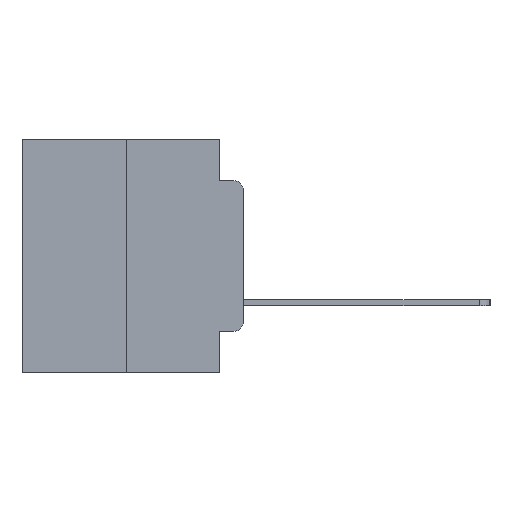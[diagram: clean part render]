
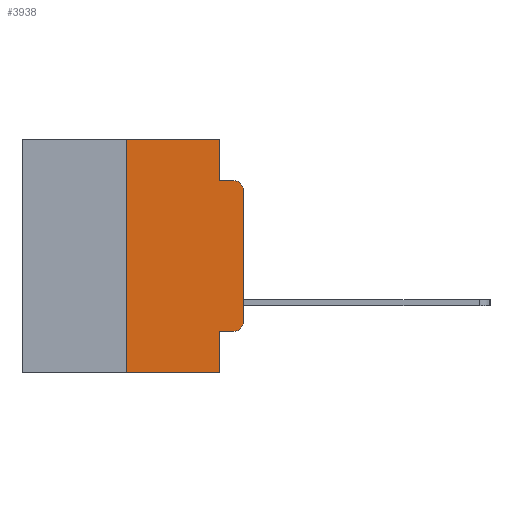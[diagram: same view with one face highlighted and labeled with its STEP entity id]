
A CAD part, left-side view. The second image highlights one B-rep face of the part: STEP entity #3938.
In plain terms, the highlighted planar face has unit normal (-1, 0, 0).
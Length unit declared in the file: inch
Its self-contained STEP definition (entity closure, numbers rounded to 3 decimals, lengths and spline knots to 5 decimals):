
#409 = DIRECTION ( 'NONE',  ( 0., 0., -1. ) ) ;
#796 = VECTOR ( 'NONE', #15762, 39.37008 ) ;
#1308 = DIRECTION ( 'NONE',  ( 0., 0., 1. ) ) ;
#1438 = DIRECTION ( 'NONE',  ( 0., -1., 0. ) ) ;
#1611 = ORIENTED_EDGE ( 'NONE', *, *, #8251, .T. ) ;
#1796 = EDGE_CURVE ( 'NONE', #16303, #14823, #22800, .T. ) ;
#1822 = AXIS2_PLACEMENT_3D ( 'NONE', #10927, #16995, #4756 ) ;
#1959 = ORIENTED_EDGE ( 'NONE', *, *, #18821, .T. ) ;
#2013 = DIRECTION ( 'NONE',  ( 0., 0., 1. ) ) ;
#2333 = DIRECTION ( 'NONE',  ( 0., -1., 0. ) ) ;
#2638 = VERTEX_POINT ( 'NONE', #8417 ) ;
#2821 = CARTESIAN_POINT ( 'NONE',  ( 0., 0.25, 0. ) ) ;
#3278 = CARTESIAN_POINT ( 'NONE',  ( 0., 0.051, -0.0885 ) ) ;
#3528 = CARTESIAN_POINT ( 'NONE',  ( 0., 0.051, -0.0885 ) ) ;
#3628 = EDGE_CURVE ( 'NONE', #17064, #21599, #8734, .T. ) ;
#3787 = EDGE_CURVE ( 'NONE', #5490, #16797, #9671, .T. ) ;
#3938 = ADVANCED_FACE ( 'NONE', ( #12511 ), #14987, .F. ) ;
#4165 = VECTOR ( 'NONE', #7035, 39.37008 ) ;
#4756 = DIRECTION ( 'NONE',  ( 0., 0., -1. ) ) ;
#5264 = ORIENTED_EDGE ( 'NONE', *, *, #3787, .T. ) ;
#5490 = VERTEX_POINT ( 'NONE', #13115 ) ;
#5694 = ORIENTED_EDGE ( 'NONE', *, *, #17550, .F. ) ;
#5700 = CARTESIAN_POINT ( 'NONE',  ( 0., 0.051, 0. ) ) ;
#5862 = LINE ( 'NONE', #12696, #10698 ) ;
#6356 = ORIENTED_EDGE ( 'NONE', *, *, #10285, .F. ) ;
#7035 = DIRECTION ( 'NONE',  ( 0., -1., 0. ) ) ;
#7657 = CARTESIAN_POINT ( 'NONE',  ( 0., 0.051, 0. ) ) ;
#8251 = EDGE_CURVE ( 'NONE', #18702, #2638, #5862, .T. ) ;
#8417 = CARTESIAN_POINT ( 'NONE',  ( 0., 0.02, -0.4115 ) ) ;
#8734 = LINE ( 'NONE', #13289, #24226 ) ;
#9098 = CARTESIAN_POINT ( 'NONE',  ( 0., 0.473, 0. ) ) ;
#9204 = CARTESIAN_POINT ( 'NONE',  ( 0., 0.25, -0.5 ) ) ;
#9342 = CARTESIAN_POINT ( 'NONE',  ( 0., 0.051, -0.4115 ) ) ;
#9671 = LINE ( 'NONE', #22636, #25134 ) ;
#9690 = DIRECTION ( 'NONE',  ( 0., 0., -1. ) ) ;
#10285 = EDGE_CURVE ( 'NONE', #24908, #16303, #22058, .T. ) ;
#10698 = VECTOR ( 'NONE', #2333, 39.37008 ) ;
#10872 = DIRECTION ( 'NONE',  ( -1., 0., 0. ) ) ;
#10927 = CARTESIAN_POINT ( 'NONE',  ( 0., 0.473, 0. ) ) ;
#10940 = CIRCLE ( 'NONE', #12037, 0.02 ) ;
#10965 = LINE ( 'NONE', #13715, #25144 ) ;
#11263 = VECTOR ( 'NONE', #409, 39.37008 ) ;
#11899 = DIRECTION ( 'NONE',  ( -1., 0., 0. ) ) ;
#12037 = AXIS2_PLACEMENT_3D ( 'NONE', #24014, #11899, #25982 ) ;
#12206 = LINE ( 'NONE', #7657, #22361 ) ;
#12511 = FACE_OUTER_BOUND ( 'NONE', #22265, .T. ) ;
#12537 = CARTESIAN_POINT ( 'NONE',  ( 0., 0.051, -0.5 ) ) ;
#12696 = CARTESIAN_POINT ( 'NONE',  ( 0., 0.051, -0.4115 ) ) ;
#13115 = CARTESIAN_POINT ( 'NONE',  ( 0., 0., -0.3915 ) ) ;
#13289 = CARTESIAN_POINT ( 'NONE',  ( 0., 0.473, -0.5 ) ) ;
#13679 = ORIENTED_EDGE ( 'NONE', *, *, #21668, .T. ) ;
#13715 = CARTESIAN_POINT ( 'NONE',  ( 0., 0.25, 0. ) ) ;
#14823 = VERTEX_POINT ( 'NONE', #25898 ) ;
#14987 = PLANE ( 'NONE',  #1822 ) ;
#15119 = LINE ( 'NONE', #9098, #4165 ) ;
#15287 = ORIENTED_EDGE ( 'NONE', *, *, #18433, .F. ) ;
#15762 = DIRECTION ( 'NONE',  ( 0., -1., 0. ) ) ;
#16303 = VERTEX_POINT ( 'NONE', #3528 ) ;
#16797 = VERTEX_POINT ( 'NONE', #25604 ) ;
#16979 = CARTESIAN_POINT ( 'NONE',  ( 0., 0.051, 0. ) ) ;
#16995 = DIRECTION ( 'NONE',  ( 1., 0., 0. ) ) ;
#17064 = VERTEX_POINT ( 'NONE', #9204 ) ;
#17550 = EDGE_CURVE ( 'NONE', #21756, #24908, #15119, .T. ) ;
#17808 = ORIENTED_EDGE ( 'NONE', *, *, #1796, .F. ) ;
#18433 = EDGE_CURVE ( 'NONE', #17064, #21756, #10965, .T. ) ;
#18702 = VERTEX_POINT ( 'NONE', #9342 ) ;
#18778 = EDGE_CURVE ( 'NONE', #18702, #21599, #12206, .T. ) ;
#18821 = EDGE_CURVE ( 'NONE', #2638, #5490, #10940, .T. ) ;
#19891 = CIRCLE ( 'NONE', #20416, 0.02 ) ;
#20416 = AXIS2_PLACEMENT_3D ( 'NONE', #23007, #10872, #24958 ) ;
#21599 = VERTEX_POINT ( 'NONE', #12537 ) ;
#21668 = EDGE_CURVE ( 'NONE', #16797, #14823, #19891, .T. ) ;
#21756 = VERTEX_POINT ( 'NONE', #2821 ) ;
#22058 = LINE ( 'NONE', #16979, #11263 ) ;
#22265 = EDGE_LOOP ( 'NONE', ( #5264, #13679, #17808, #6356, #5694, #15287, #25064, #23506, #1611, #1959 ) ) ;
#22361 = VECTOR ( 'NONE', #9690, 39.37008 ) ;
#22636 = CARTESIAN_POINT ( 'NONE',  ( 0., 0., 0. ) ) ;
#22800 = LINE ( 'NONE', #3278, #796 ) ;
#23007 = CARTESIAN_POINT ( 'NONE',  ( 0., 0.02, -0.1085 ) ) ;
#23506 = ORIENTED_EDGE ( 'NONE', *, *, #18778, .F. ) ;
#24014 = CARTESIAN_POINT ( 'NONE',  ( 0., 0.02, -0.3915 ) ) ;
#24226 = VECTOR ( 'NONE', #1438, 39.37008 ) ;
#24908 = VERTEX_POINT ( 'NONE', #5700 ) ;
#24958 = DIRECTION ( 'NONE',  ( 0., 0., -1. ) ) ;
#25064 = ORIENTED_EDGE ( 'NONE', *, *, #3628, .T. ) ;
#25134 = VECTOR ( 'NONE', #2013, 39.37008 ) ;
#25144 = VECTOR ( 'NONE', #1308, 39.37008 ) ;
#25604 = CARTESIAN_POINT ( 'NONE',  ( 0., 0., -0.1085 ) ) ;
#25898 = CARTESIAN_POINT ( 'NONE',  ( 0., 0.02, -0.0885 ) ) ;
#25982 = DIRECTION ( 'NONE',  ( 0., 0., -1. ) ) ;
